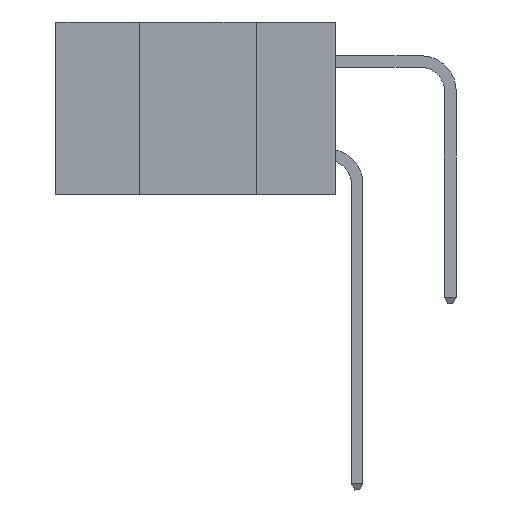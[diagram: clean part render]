
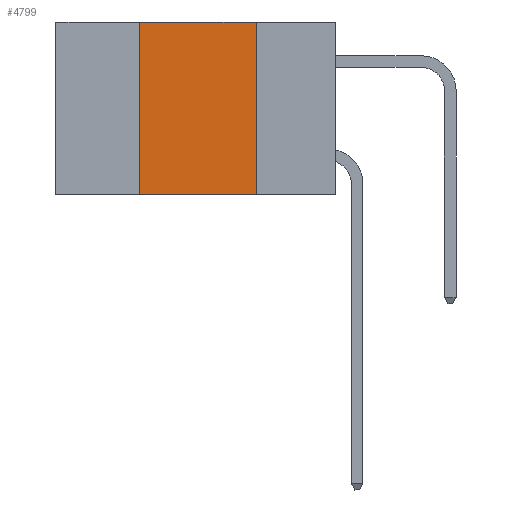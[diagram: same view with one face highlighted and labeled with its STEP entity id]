
A CAD part, left-side view. The second image highlights one B-rep face of the part: STEP entity #4799.
In plain terms, the highlighted planar face has unit normal (-1, 0, 0).
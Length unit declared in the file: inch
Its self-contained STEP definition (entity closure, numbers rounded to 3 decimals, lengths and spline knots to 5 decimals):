
#1156 = FACE_OUTER_BOUND ( 'NONE', #21368, .T. ) ;
#2779 = EDGE_CURVE ( 'NONE', #18688, #29603, #17540, .T. ) ;
#4116 = ORIENTED_EDGE ( 'NONE', *, *, #8621, .F. ) ;
#4799 = ADVANCED_FACE ( 'NONE', ( #1156 ), #19217, .F. ) ;
#6563 = DIRECTION ( 'NONE',  ( 0., -1., 0. ) ) ;
#6896 = CARTESIAN_POINT ( 'NONE',  ( 0., 0.17, 0. ) ) ;
#8621 = EDGE_CURVE ( 'NONE', #20159, #11955, #28061, .T. ) ;
#8854 = CARTESIAN_POINT ( 'NONE',  ( 0., 0.42, 0. ) ) ;
#8971 = LINE ( 'NONE', #11213, #29445 ) ;
#9814 = CARTESIAN_POINT ( 'NONE',  ( 0., 0.17, 0. ) ) ;
#10007 = VECTOR ( 'NONE', #29546, 39.37008 ) ;
#10804 = ORIENTED_EDGE ( 'NONE', *, *, #27468, .T. ) ;
#11213 = CARTESIAN_POINT ( 'NONE',  ( 0., 0.6, 0. ) ) ;
#11638 = CARTESIAN_POINT ( 'NONE',  ( 0., 0.6, 0. ) ) ;
#11955 = VERTEX_POINT ( 'NONE', #8854 ) ;
#13493 = VECTOR ( 'NONE', #27812, 39.37008 ) ;
#13653 = LINE ( 'NONE', #14151, #10007 ) ;
#14001 = VECTOR ( 'NONE', #14385, 39.37008 ) ;
#14062 = DIRECTION ( 'NONE',  ( 0., 0., -1. ) ) ;
#14151 = CARTESIAN_POINT ( 'NONE',  ( 0., 0.6, -0.37 ) ) ;
#14385 = DIRECTION ( 'NONE',  ( 0., 0., 1. ) ) ;
#16480 = EDGE_CURVE ( 'NONE', #11955, #18688, #8971, .T. ) ;
#17540 = LINE ( 'NONE', #9814, #13493 ) ;
#18688 = VERTEX_POINT ( 'NONE', #6896 ) ;
#18738 = CARTESIAN_POINT ( 'NONE',  ( 0., 0.42, -0.37 ) ) ;
#19217 = PLANE ( 'NONE',  #31341 ) ;
#20159 = VERTEX_POINT ( 'NONE', #18738 ) ;
#21368 = EDGE_LOOP ( 'NONE', ( #28821, #27906, #4116, #10804 ) ) ;
#22940 = CARTESIAN_POINT ( 'NONE',  ( 0., 0.42, 0. ) ) ;
#27468 = EDGE_CURVE ( 'NONE', #20159, #29603, #13653, .T. ) ;
#27812 = DIRECTION ( 'NONE',  ( 0., 0., -1. ) ) ;
#27906 = ORIENTED_EDGE ( 'NONE', *, *, #16480, .F. ) ;
#28061 = LINE ( 'NONE', #22940, #14001 ) ;
#28473 = CARTESIAN_POINT ( 'NONE',  ( 0., 0.17, -0.37 ) ) ;
#28821 = ORIENTED_EDGE ( 'NONE', *, *, #2779, .F. ) ;
#29445 = VECTOR ( 'NONE', #6563, 39.37008 ) ;
#29546 = DIRECTION ( 'NONE',  ( 0., -1., 0. ) ) ;
#29603 = VERTEX_POINT ( 'NONE', #28473 ) ;
#29963 = DIRECTION ( 'NONE',  ( 1., 0., 0. ) ) ;
#31341 = AXIS2_PLACEMENT_3D ( 'NONE', #11638, #29963, #14062 ) ;
